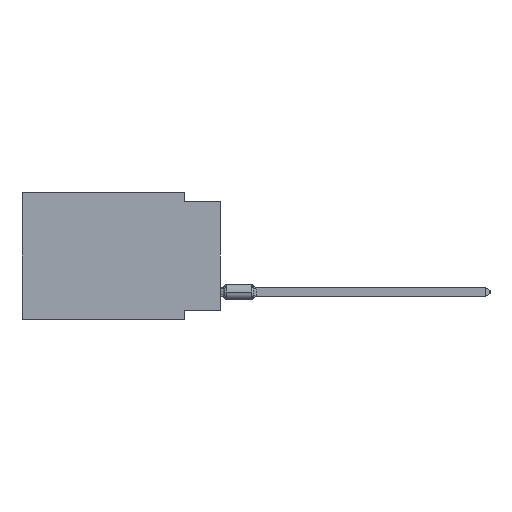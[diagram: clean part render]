
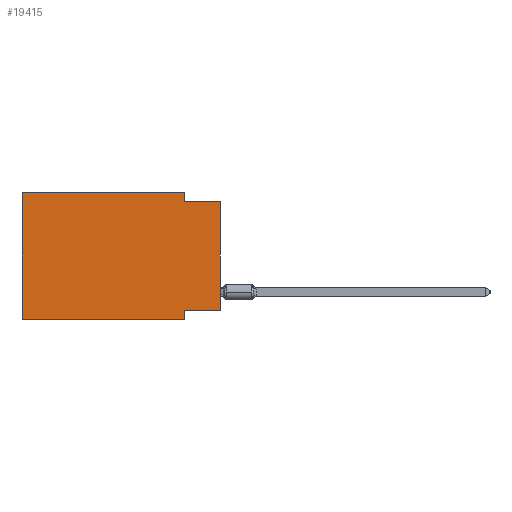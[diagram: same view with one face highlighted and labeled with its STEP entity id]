
A CAD part, left-side view. The second image highlights one B-rep face of the part: STEP entity #19415.
In plain terms, the highlighted planar face has unit normal (-1, 0, 0).
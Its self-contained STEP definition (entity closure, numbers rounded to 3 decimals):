
#1271 = DIRECTION ( 'NONE',  ( 0., 0., -1. ) ) ;
#1336 = DIRECTION ( 'NONE',  ( 0., 0., -1. ) ) ;
#1661 = EDGE_CURVE ( 'NONE', #50310, #38898, #51460, .T. ) ;
#1837 = ORIENTED_EDGE ( 'NONE', *, *, #17893, .F. ) ;
#2136 = DIRECTION ( 'NONE',  ( 0., 0., -1. ) ) ;
#2903 = VERTEX_POINT ( 'NONE', #47406 ) ;
#4233 = CARTESIAN_POINT ( 'NONE',  ( 0., 0., -0.635 ) ) ;
#5387 = EDGE_LOOP ( 'NONE', ( #11592, #8784, #31617, #10532, #23599, #38032, #43494, #1837 ) ) ;
#5548 = FACE_OUTER_BOUND ( 'NONE', #5387, .T. ) ;
#8478 = DIRECTION ( 'NONE',  ( 0., -1., 0. ) ) ;
#8784 = ORIENTED_EDGE ( 'NONE', *, *, #28656, .F. ) ;
#10532 = ORIENTED_EDGE ( 'NONE', *, *, #51986, .F. ) ;
#11167 = VERTEX_POINT ( 'NONE', #27823 ) ;
#11363 = LINE ( 'NONE', #19771, #33640 ) ;
#11592 = ORIENTED_EDGE ( 'NONE', *, *, #43476, .T. ) ;
#13199 = LINE ( 'NONE', #25752, #51469 ) ;
#13241 = DIRECTION ( 'NONE',  ( 0., -1., 0. ) ) ;
#13520 = CARTESIAN_POINT ( 'NONE',  ( 0., 13.97, -8.89 ) ) ;
#15415 = VERTEX_POINT ( 'NONE', #40970 ) ;
#17594 = VECTOR ( 'NONE', #36937, 1000. ) ;
#17893 = EDGE_CURVE ( 'NONE', #11167, #15415, #11363, .T. ) ;
#18101 = EDGE_CURVE ( 'NONE', #41467, #52941, #26690, .T. ) ;
#19415 = ADVANCED_FACE ( 'NONE', ( #5548 ), #44289, .F. ) ;
#19771 = CARTESIAN_POINT ( 'NONE',  ( 0., 0., -8.255 ) ) ;
#21244 = LINE ( 'NONE', #28799, #35832 ) ;
#22583 = CARTESIAN_POINT ( 'NONE',  ( 0., 13.97, 0. ) ) ;
#23369 = LINE ( 'NONE', #40387, #36557 ) ;
#23599 = ORIENTED_EDGE ( 'NONE', *, *, #39831, .F. ) ;
#25752 = CARTESIAN_POINT ( 'NONE',  ( 0., 13.97, 0. ) ) ;
#26690 = LINE ( 'NONE', #39770, #37228 ) ;
#26951 = CARTESIAN_POINT ( 'NONE',  ( 0., 13.97, 0. ) ) ;
#27823 = CARTESIAN_POINT ( 'NONE',  ( 0., 0., -8.255 ) ) ;
#28656 = EDGE_CURVE ( 'NONE', #52941, #2903, #30187, .T. ) ;
#28799 = CARTESIAN_POINT ( 'NONE',  ( 0., 0., 0. ) ) ;
#29661 = EDGE_CURVE ( 'NONE', #15415, #38898, #23369, .T. ) ;
#30187 = LINE ( 'NONE', #4233, #45284 ) ;
#31044 = CARTESIAN_POINT ( 'NONE',  ( 0., 2.54, -8.89 ) ) ;
#31617 = ORIENTED_EDGE ( 'NONE', *, *, #18101, .F. ) ;
#33640 = VECTOR ( 'NONE', #49868, 1000. ) ;
#33840 = DIRECTION ( 'NONE',  ( 0., -1., 0. ) ) ;
#35346 = VERTEX_POINT ( 'NONE', #26951 ) ;
#35832 = VECTOR ( 'NONE', #54458, 1000. ) ;
#36121 = LINE ( 'NONE', #36668, #17594 ) ;
#36557 = VECTOR ( 'NONE', #2136, 1000. ) ;
#36668 = CARTESIAN_POINT ( 'NONE',  ( 0., 13.97, 0. ) ) ;
#36937 = DIRECTION ( 'NONE',  ( 0., 0., 1. ) ) ;
#37228 = VECTOR ( 'NONE', #1271, 1000. ) ;
#38032 = ORIENTED_EDGE ( 'NONE', *, *, #1661, .T. ) ;
#38898 = VERTEX_POINT ( 'NONE', #31044 ) ;
#39292 = CARTESIAN_POINT ( 'NONE',  ( 0., 13.97, -8.89 ) ) ;
#39579 = DIRECTION ( 'NONE',  ( 1., 0., 0. ) ) ;
#39770 = CARTESIAN_POINT ( 'NONE',  ( 0., 2.54, 0. ) ) ;
#39831 = EDGE_CURVE ( 'NONE', #50310, #35346, #36121, .T. ) ;
#40040 = VECTOR ( 'NONE', #13241, 1000. ) ;
#40387 = CARTESIAN_POINT ( 'NONE',  ( 0., 2.54, -8.89 ) ) ;
#40970 = CARTESIAN_POINT ( 'NONE',  ( 0., 2.54, -8.255 ) ) ;
#41467 = VERTEX_POINT ( 'NONE', #50378 ) ;
#43476 = EDGE_CURVE ( 'NONE', #11167, #2903, #21244, .T. ) ;
#43494 = ORIENTED_EDGE ( 'NONE', *, *, #29661, .F. ) ;
#44289 = PLANE ( 'NONE',  #47177 ) ;
#45284 = VECTOR ( 'NONE', #33840, 1000. ) ;
#47177 = AXIS2_PLACEMENT_3D ( 'NONE', #22583, #39579, #1336 ) ;
#47406 = CARTESIAN_POINT ( 'NONE',  ( 0., 0., -0.635 ) ) ;
#49868 = DIRECTION ( 'NONE',  ( 0., 1., 0. ) ) ;
#50310 = VERTEX_POINT ( 'NONE', #39292 ) ;
#50378 = CARTESIAN_POINT ( 'NONE',  ( 0., 2.54, 0. ) ) ;
#51460 = LINE ( 'NONE', #13520, #40040 ) ;
#51469 = VECTOR ( 'NONE', #8478, 1000. ) ;
#51986 = EDGE_CURVE ( 'NONE', #35346, #41467, #13199, .T. ) ;
#52890 = CARTESIAN_POINT ( 'NONE',  ( 0., 2.54, -0.635 ) ) ;
#52941 = VERTEX_POINT ( 'NONE', #52890 ) ;
#54458 = DIRECTION ( 'NONE',  ( 0., 0., 1. ) ) ;
